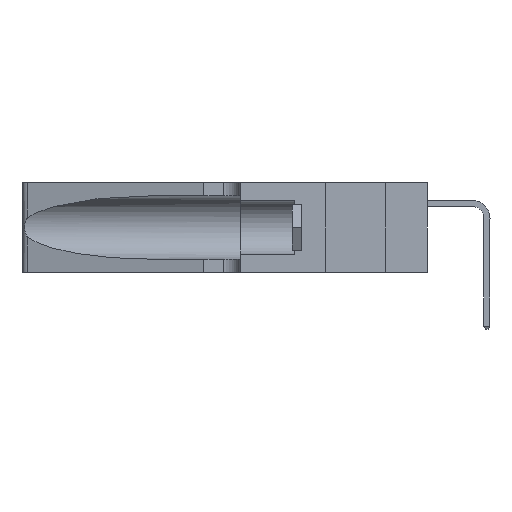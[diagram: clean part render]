
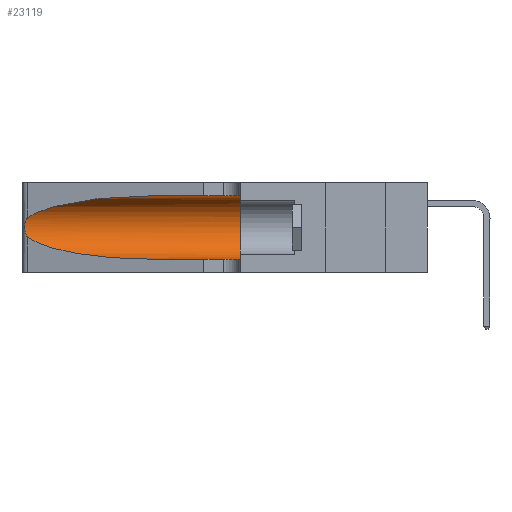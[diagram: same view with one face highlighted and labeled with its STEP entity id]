
A CAD part, left-side view. The second image highlights one B-rep face of the part: STEP entity #23119.
In plain terms, the highlighted cylindrical face has radius 3.308 mm (diameter 6.617 mm), a partial arc.
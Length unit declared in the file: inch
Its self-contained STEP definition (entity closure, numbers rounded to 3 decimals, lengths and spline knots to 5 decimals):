
#27 = CARTESIAN_POINT ( 'NONE',  ( 0.1305, 0.72297, 0.05475 ) ) ;
#700 = CARTESIAN_POINT ( 'NONE',  ( 0.1305, 1.61858, 0.05475 ) ) ;
#939 = AXIS2_PLACEMENT_3D ( 'NONE', #5535, #26223, #34978 ) ;
#1988 = CARTESIAN_POINT ( 'NONE',  ( 0.25854, 1.2359, 0.20912 ) ) ;
#3125 = CARTESIAN_POINT ( 'NONE',  ( 0.1305, 0.35, 0.31525 ) ) ;
#4730 = VERTEX_POINT ( 'NONE', #29922 ) ;
#5010 = CARTESIAN_POINT ( 'NONE',  ( 0.26075, 1.23896, 0.19203 ) ) ;
#5535 = CARTESIAN_POINT ( 'NONE',  ( 0.1305, 1.61858, 0.185 ) ) ;
#5830 = VERTEX_POINT ( 'NONE', #20123 ) ;
#6389 = CARTESIAN_POINT ( 'NONE',  ( 0.1305, 0.72297, 0.31525 ) ) ;
#7318 = VERTEX_POINT ( 'NONE', #6389 ) ;
#8087 = CARTESIAN_POINT ( 'NONE',  ( 0.26017, 1.23833, 0.17102 ) ) ;
#8168 = VECTOR ( 'NONE', #33608, 39.37008 ) ;
#8624 =( BOUNDED_CURVE ( )  B_SPLINE_CURVE ( 3, ( #35502, #15028, #17956, #27 ),
 .UNSPECIFIED., .F., .F. ) 
 B_SPLINE_CURVE_WITH_KNOTS ( ( 4, 4 ),
 ( 3.44316, 4.71239 ),
 .UNSPECIFIED. ) 
 CURVE ( )  GEOMETRIC_REPRESENTATION_ITEM ( )  RATIONAL_B_SPLINE_CURVE ( ( 1., 0.87, 0.87, 1. ) ) 
 REPRESENTATION_ITEM ( '' )  );
#9014 = CARTESIAN_POINT ( 'NONE',  ( 0.18966, 0.96281, 0.31525 ) ) ;
#9481 = AXIS2_PLACEMENT_3D ( 'NONE', #27143, #9531, #30080 ) ;
#9521 = CARTESIAN_POINT ( 'NONE',  ( 0.1305, 0.35, 0.05475 ) ) ;
#9531 = DIRECTION ( 'NONE',  ( 0., 1., 0. ) ) ;
#10104 = CARTESIAN_POINT ( 'NONE',  ( 0.1305, 1.61858, 0.31525 ) ) ;
#11068 = CARTESIAN_POINT ( 'NONE',  ( 0.25789, 1.23486, 0.15765 ) ) ;
#12809 = EDGE_LOOP ( 'NONE', ( #22407, #16822, #14545, #25818, #15112, #33525 ) ) ;
#13143 =( BOUNDED_CURVE ( )  B_SPLINE_CURVE ( 3, ( #29564, #9014, #32551, #15032 ),
 .UNSPECIFIED., .F., .T. ) 
 B_SPLINE_CURVE_WITH_KNOTS ( ( 4, 4 ),
 ( 1.5708, 2.84003 ),
 .UNSPECIFIED. ) 
 CURVE ( )  GEOMETRIC_REPRESENTATION_ITEM ( )  RATIONAL_B_SPLINE_CURVE ( ( 1., 0.87, 0.87, 1. ) ) 
 REPRESENTATION_ITEM ( '' )  );
#13963 = CARTESIAN_POINT ( 'NONE',  ( 0.25555, 1.22994, 0.2215 ) ) ;
#14074 = CARTESIAN_POINT ( 'NONE',  ( 0.25555, 1.22993, 0.14849 ) ) ;
#14144 = EDGE_CURVE ( 'NONE', #5830, #4730, #8624, .T. ) ;
#14426 = FACE_OUTER_BOUND ( 'NONE', #12809, .T. ) ;
#14545 = ORIENTED_EDGE ( 'NONE', *, *, #14144, .T. ) ;
#15028 = CARTESIAN_POINT ( 'NONE',  ( 0.2373, 1.15595, 0.08982 ) ) ;
#15032 = CARTESIAN_POINT ( 'NONE',  ( 0.25487, 1.22718, 0.22369 ) ) ;
#15112 = ORIENTED_EDGE ( 'NONE', *, *, #21146, .F. ) ;
#15550 = EDGE_CURVE ( 'NONE', #7318, #31094, #31624, .T. ) ;
#16822 = ORIENTED_EDGE ( 'NONE', *, *, #35931, .T. ) ;
#17956 = CARTESIAN_POINT ( 'NONE',  ( 0.18966, 0.96281, 0.05475 ) ) ;
#18719 = DIRECTION ( 'NONE',  ( 0., -1., 0. ) ) ;
#18779 = EDGE_CURVE ( 'NONE', #7318, #36296, #13143, .T. ) ;
#19849 = CARTESIAN_POINT ( 'NONE',  ( 0.25787, 1.23484, 0.2124 ) ) ;
#20123 = CARTESIAN_POINT ( 'NONE',  ( 0.25487, 1.22718, 0.14631 ) ) ;
#20695 = VECTOR ( 'NONE', #18719, 39.37008 ) ;
#21146 = EDGE_CURVE ( 'NONE', #31094, #29989, #23722, .T. ) ;
#22407 = ORIENTED_EDGE ( 'NONE', *, *, #18779, .T. ) ;
#22803 = CARTESIAN_POINT ( 'NONE',  ( 0.26018, 1.23835, 0.19895 ) ) ;
#23119 = ADVANCED_FACE ( 'NONE', ( #14426 ), #29033, .F. ) ;
#23722 = CIRCLE ( 'NONE', #9481, 0.13025 ) ;
#24533 = EDGE_CURVE ( 'NONE', #4730, #29989, #28458, .T. ) ;
#25694 = CARTESIAN_POINT ( 'NONE',  ( 0.26075, 1.23896, 0.178 ) ) ;
#25818 = ORIENTED_EDGE ( 'NONE', *, *, #24533, .T. ) ;
#26223 = DIRECTION ( 'NONE',  ( 0., -1., 0. ) ) ;
#27143 = CARTESIAN_POINT ( 'NONE',  ( 0.1305, 0.35, 0.185 ) ) ;
#28458 = LINE ( 'NONE', #700, #20695 ) ;
#28513 = CARTESIAN_POINT ( 'NONE',  ( 0.25487, 1.22718, 0.22369 ) ) ;
#28638 = CARTESIAN_POINT ( 'NONE',  ( 0.25856, 1.23593, 0.16098 ) ) ;
#29033 = CYLINDRICAL_SURFACE ( 'NONE', #939, 0.13025 ) ;
#29564 = CARTESIAN_POINT ( 'NONE',  ( 0.1305, 0.72297, 0.31525 ) ) ;
#29922 = CARTESIAN_POINT ( 'NONE',  ( 0.1305, 0.72297, 0.05475 ) ) ;
#29989 = VERTEX_POINT ( 'NONE', #9521 ) ;
#30058 = B_SPLINE_CURVE_WITH_KNOTS ( 'NONE', 3,
 ( #28513, #13963, #37400, #19849, #1988, #22803, #5010, #25694, #8087, #28638, #11068, #31607, #14074, #34563 ),
 .UNSPECIFIED., .F., .F.,
 ( 4, 2, 2, 2, 2, 2, 4 ),
 ( 0., 0.00027, 0.00053, 0.00107, 0.0016, 0.00187, 0.00214 ),
 .UNSPECIFIED. ) ;
#30080 = DIRECTION ( 'NONE',  ( 0., 0., 1. ) ) ;
#31094 = VERTEX_POINT ( 'NONE', #3125 ) ;
#31607 = CARTESIAN_POINT ( 'NONE',  ( 0.25639, 1.23186, 0.15144 ) ) ;
#31624 = LINE ( 'NONE', #10104, #8168 ) ;
#32551 = CARTESIAN_POINT ( 'NONE',  ( 0.2373, 1.15595, 0.28018 ) ) ;
#33525 = ORIENTED_EDGE ( 'NONE', *, *, #15550, .F. ) ;
#33608 = DIRECTION ( 'NONE',  ( 0., -1., 0. ) ) ;
#34563 = CARTESIAN_POINT ( 'NONE',  ( 0.25487, 1.22718, 0.14631 ) ) ;
#34978 = DIRECTION ( 'NONE',  ( 0., 0., -1. ) ) ;
#35502 = CARTESIAN_POINT ( 'NONE',  ( 0.25487, 1.22718, 0.14631 ) ) ;
#35931 = EDGE_CURVE ( 'NONE', #36296, #5830, #30058, .T. ) ;
#36202 = CARTESIAN_POINT ( 'NONE',  ( 0.25487, 1.22718, 0.22369 ) ) ;
#36296 = VERTEX_POINT ( 'NONE', #36202 ) ;
#37400 = CARTESIAN_POINT ( 'NONE',  ( 0.25639, 1.23184, 0.21858 ) ) ;
